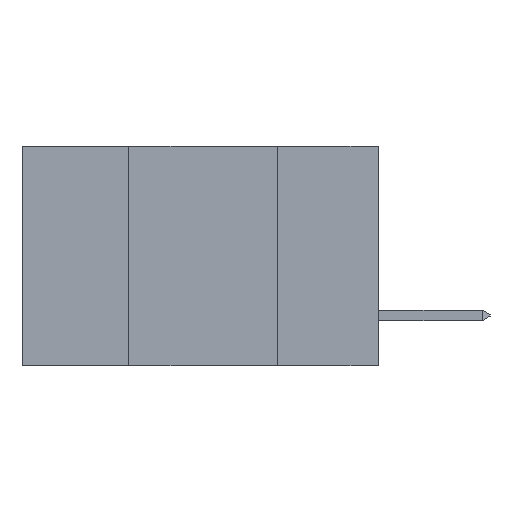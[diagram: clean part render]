
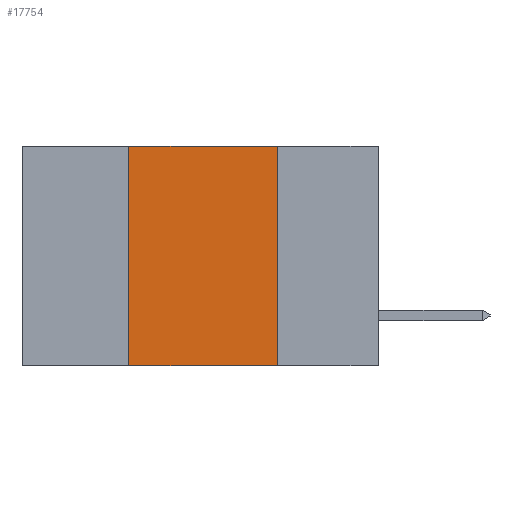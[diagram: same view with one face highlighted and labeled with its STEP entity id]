
A CAD part, left-side view. The second image highlights one B-rep face of the part: STEP entity #17754.
In plain terms, the highlighted planar face has unit normal (-1, 0, 0).
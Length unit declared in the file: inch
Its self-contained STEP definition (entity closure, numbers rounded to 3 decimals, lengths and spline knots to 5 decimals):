
#1033 = EDGE_CURVE ( 'NONE', #16209, #2054, #13723, .T. ) ;
#1161 = DIRECTION ( 'NONE',  ( 0., 0., -1. ) ) ;
#1369 = ORIENTED_EDGE ( 'NONE', *, *, #1033, .F. ) ;
#1631 = VECTOR ( 'NONE', #9822, 39.37008 ) ;
#2054 = VERTEX_POINT ( 'NONE', #8528 ) ;
#2864 = LINE ( 'NONE', #17401, #6230 ) ;
#5067 = DIRECTION ( 'NONE',  ( 0., -1., 0. ) ) ;
#5911 = VERTEX_POINT ( 'NONE', #6809 ) ;
#5922 = LINE ( 'NONE', #8439, #1631 ) ;
#6230 = VECTOR ( 'NONE', #5067, 39.37008 ) ;
#6432 = CARTESIAN_POINT ( 'NONE',  ( 0., 0.17, 0. ) ) ;
#6664 = DIRECTION ( 'NONE',  ( 0., 0., -1. ) ) ;
#6809 = CARTESIAN_POINT ( 'NONE',  ( 0., 0.42, -0.37 ) ) ;
#7577 = FACE_OUTER_BOUND ( 'NONE', #11608, .T. ) ;
#8439 = CARTESIAN_POINT ( 'NONE',  ( 0., 0.42, 0. ) ) ;
#8528 = CARTESIAN_POINT ( 'NONE',  ( 0., 0.17, -0.37 ) ) ;
#8898 = ORIENTED_EDGE ( 'NONE', *, *, #11157, .F. ) ;
#8965 = AXIS2_PLACEMENT_3D ( 'NONE', #12351, #9607, #1161 ) ;
#9258 = CARTESIAN_POINT ( 'NONE',  ( 0., 0.17, 0. ) ) ;
#9333 = ORIENTED_EDGE ( 'NONE', *, *, #9884, .T. ) ;
#9607 = DIRECTION ( 'NONE',  ( 1., 0., 0. ) ) ;
#9609 = VECTOR ( 'NONE', #6664, 39.37008 ) ;
#9822 = DIRECTION ( 'NONE',  ( 0., 0., 1. ) ) ;
#9884 = EDGE_CURVE ( 'NONE', #5911, #2054, #17418, .T. ) ;
#11157 = EDGE_CURVE ( 'NONE', #14589, #16209, #2864, .T. ) ;
#11425 = DIRECTION ( 'NONE',  ( 0., -1., 0. ) ) ;
#11498 = ORIENTED_EDGE ( 'NONE', *, *, #13599, .F. ) ;
#11608 = EDGE_LOOP ( 'NONE', ( #1369, #8898, #11498, #9333 ) ) ;
#12351 = CARTESIAN_POINT ( 'NONE',  ( 0., 0.6, 0. ) ) ;
#12769 = CARTESIAN_POINT ( 'NONE',  ( 0., 0.6, -0.37 ) ) ;
#13599 = EDGE_CURVE ( 'NONE', #5911, #14589, #5922, .T. ) ;
#13723 = LINE ( 'NONE', #6432, #9609 ) ;
#13881 = VECTOR ( 'NONE', #11425, 39.37008 ) ;
#14369 = CARTESIAN_POINT ( 'NONE',  ( 0., 0.42, 0. ) ) ;
#14589 = VERTEX_POINT ( 'NONE', #14369 ) ;
#16209 = VERTEX_POINT ( 'NONE', #9258 ) ;
#17401 = CARTESIAN_POINT ( 'NONE',  ( 0., 0.6, 0. ) ) ;
#17418 = LINE ( 'NONE', #12769, #13881 ) ;
#17719 = PLANE ( 'NONE',  #8965 ) ;
#17754 = ADVANCED_FACE ( 'NONE', ( #7577 ), #17719, .F. ) ;
